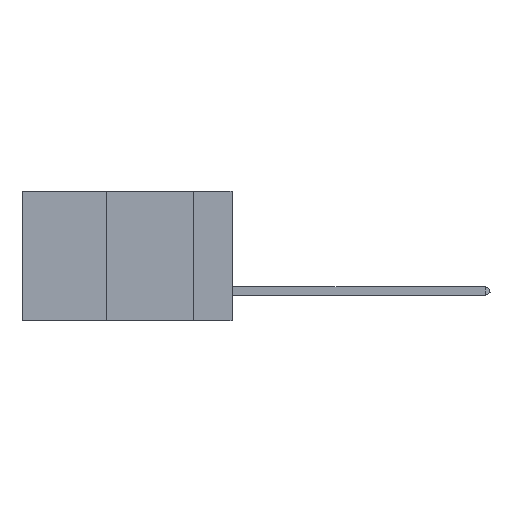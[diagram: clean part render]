
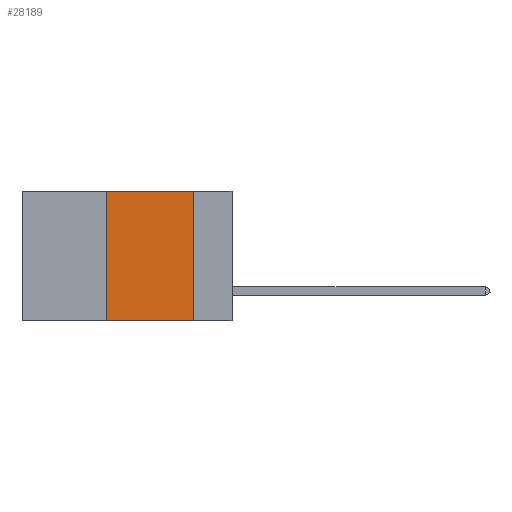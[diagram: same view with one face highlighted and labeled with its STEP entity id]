
A CAD part, left-side view. The second image highlights one B-rep face of the part: STEP entity #28189.
In plain terms, the highlighted planar face has unit normal (-1, 0, 0).
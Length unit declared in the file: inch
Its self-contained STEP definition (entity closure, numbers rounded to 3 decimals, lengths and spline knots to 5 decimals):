
#120 = CARTESIAN_POINT ( 'NONE',  ( 0., 0.11, -0.37 ) ) ;
#2108 = VERTEX_POINT ( 'NONE', #17983 ) ;
#5806 = CARTESIAN_POINT ( 'NONE',  ( 0., 0.11, 0. ) ) ;
#5943 = VECTOR ( 'NONE', #27646, 39.37008 ) ;
#9182 = VECTOR ( 'NONE', #25347, 39.37008 ) ;
#12260 = CARTESIAN_POINT ( 'NONE',  ( 0., 0.6, 0. ) ) ;
#12765 = VECTOR ( 'NONE', #17671, 39.37008 ) ;
#17157 = CARTESIAN_POINT ( 'NONE',  ( 0., 0.36, 0. ) ) ;
#17671 = DIRECTION ( 'NONE',  ( 0., 0., 1. ) ) ;
#17745 = ORIENTED_EDGE ( 'NONE', *, *, #31735, .T. ) ;
#17983 = CARTESIAN_POINT ( 'NONE',  ( 0., 0.11, 0. ) ) ;
#19099 = LINE ( 'NONE', #25503, #9182 ) ;
#23318 = CARTESIAN_POINT ( 'NONE',  ( 0., 0.6, 0. ) ) ;
#23473 = DIRECTION ( 'NONE',  ( 1., 0., 0. ) ) ;
#24366 = CARTESIAN_POINT ( 'NONE',  ( 0., 0.36, -0.37 ) ) ;
#24951 = EDGE_CURVE ( 'NONE', #30190, #42425, #30822, .T. ) ;
#25347 = DIRECTION ( 'NONE',  ( 0., -1., 0. ) ) ;
#25503 = CARTESIAN_POINT ( 'NONE',  ( 0., 0.6, -0.37 ) ) ;
#25759 = LINE ( 'NONE', #5806, #5943 ) ;
#26333 = EDGE_CURVE ( 'NONE', #42425, #2108, #26585, .T. ) ;
#26585 = LINE ( 'NONE', #12260, #31313 ) ;
#27646 = DIRECTION ( 'NONE',  ( 0., 0., -1. ) ) ;
#28189 = ADVANCED_FACE ( 'NONE', ( #33967 ), #45580, .F. ) ;
#28731 = EDGE_LOOP ( 'NONE', ( #30075, #48119, #29301, #17745 ) ) ;
#29301 = ORIENTED_EDGE ( 'NONE', *, *, #24951, .F. ) ;
#30075 = ORIENTED_EDGE ( 'NONE', *, *, #39299, .F. ) ;
#30190 = VERTEX_POINT ( 'NONE', #24366 ) ;
#30822 = LINE ( 'NONE', #40135, #12765 ) ;
#31313 = VECTOR ( 'NONE', #38014, 39.37008 ) ;
#31735 = EDGE_CURVE ( 'NONE', #30190, #42880, #19099, .T. ) ;
#33967 = FACE_OUTER_BOUND ( 'NONE', #28731, .T. ) ;
#37970 = DIRECTION ( 'NONE',  ( 0., 0., -1. ) ) ;
#38014 = DIRECTION ( 'NONE',  ( 0., -1., 0. ) ) ;
#39299 = EDGE_CURVE ( 'NONE', #2108, #42880, #25759, .T. ) ;
#40135 = CARTESIAN_POINT ( 'NONE',  ( 0., 0.36, 0. ) ) ;
#42425 = VERTEX_POINT ( 'NONE', #17157 ) ;
#42880 = VERTEX_POINT ( 'NONE', #120 ) ;
#45580 = PLANE ( 'NONE',  #46085 ) ;
#46085 = AXIS2_PLACEMENT_3D ( 'NONE', #23318, #23473, #37970 ) ;
#48119 = ORIENTED_EDGE ( 'NONE', *, *, #26333, .F. ) ;
